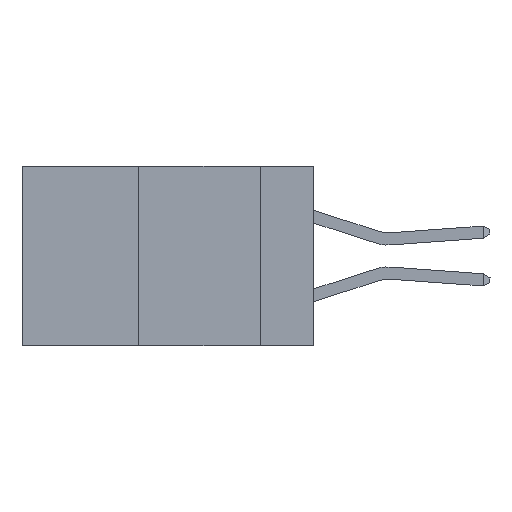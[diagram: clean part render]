
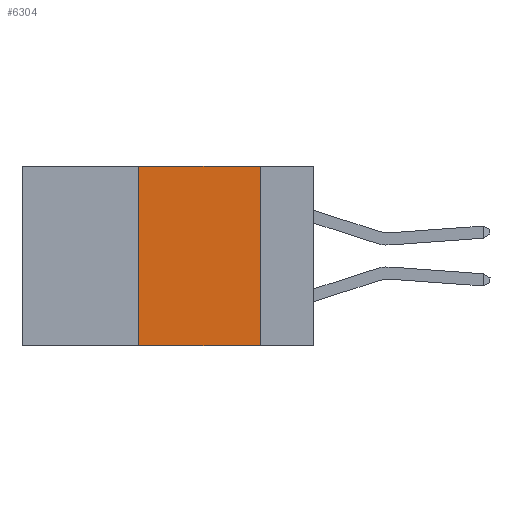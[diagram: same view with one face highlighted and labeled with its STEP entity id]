
A CAD part, left-side view. The second image highlights one B-rep face of the part: STEP entity #6304.
In plain terms, the highlighted planar face has unit normal (-1, 0, 0).
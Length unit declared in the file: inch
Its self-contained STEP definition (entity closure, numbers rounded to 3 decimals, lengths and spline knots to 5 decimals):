
#438 = DIRECTION ( 'NONE',  ( 0., -1., 0. ) ) ;
#831 = CARTESIAN_POINT ( 'NONE',  ( 0., 0.36, -0.37 ) ) ;
#860 = CARTESIAN_POINT ( 'NONE',  ( 0., 0.11, 0. ) ) ;
#1111 = CARTESIAN_POINT ( 'NONE',  ( 0., 0.36, 0. ) ) ;
#1325 = EDGE_CURVE ( 'NONE', #8755, #4644, #7580, .T. ) ;
#1890 = DIRECTION ( 'NONE',  ( 0., 0., 1. ) ) ;
#1956 = VECTOR ( 'NONE', #3213, 39.37008 ) ;
#1985 = CARTESIAN_POINT ( 'NONE',  ( 0., 0.6, -0.37 ) ) ;
#2091 = PLANE ( 'NONE',  #4279 ) ;
#2869 = LINE ( 'NONE', #1985, #8856 ) ;
#3213 = DIRECTION ( 'NONE',  ( 0., 0., -1. ) ) ;
#3431 = VECTOR ( 'NONE', #6434, 39.37008 ) ;
#3619 = ORIENTED_EDGE ( 'NONE', *, *, #7674, .F. ) ;
#3677 = DIRECTION ( 'NONE',  ( 0., 0., -1. ) ) ;
#3776 = CARTESIAN_POINT ( 'NONE',  ( 0., 0.11, 0. ) ) ;
#4201 = CARTESIAN_POINT ( 'NONE',  ( 0., 0.36, 0. ) ) ;
#4279 = AXIS2_PLACEMENT_3D ( 'NONE', #9880, #4387, #3677 ) ;
#4387 = DIRECTION ( 'NONE',  ( 1., 0., 0. ) ) ;
#4644 = VERTEX_POINT ( 'NONE', #1111 ) ;
#4693 = EDGE_CURVE ( 'NONE', #8755, #7034, #2869, .T. ) ;
#6079 = LINE ( 'NONE', #860, #1956 ) ;
#6304 = ADVANCED_FACE ( 'NONE', ( #8097 ), #2091, .F. ) ;
#6434 = DIRECTION ( 'NONE',  ( 0., -1., 0. ) ) ;
#7034 = VERTEX_POINT ( 'NONE', #9373 ) ;
#7105 = CARTESIAN_POINT ( 'NONE',  ( 0., 0.6, 0. ) ) ;
#7417 = EDGE_LOOP ( 'NONE', ( #9741, #3619, #7786, #8228 ) ) ;
#7464 = EDGE_CURVE ( 'NONE', #9459, #7034, #6079, .T. ) ;
#7580 = LINE ( 'NONE', #4201, #10023 ) ;
#7674 = EDGE_CURVE ( 'NONE', #4644, #9459, #8679, .T. ) ;
#7786 = ORIENTED_EDGE ( 'NONE', *, *, #1325, .F. ) ;
#8097 = FACE_OUTER_BOUND ( 'NONE', #7417, .T. ) ;
#8228 = ORIENTED_EDGE ( 'NONE', *, *, #4693, .T. ) ;
#8679 = LINE ( 'NONE', #7105, #3431 ) ;
#8755 = VERTEX_POINT ( 'NONE', #831 ) ;
#8856 = VECTOR ( 'NONE', #438, 39.37008 ) ;
#9373 = CARTESIAN_POINT ( 'NONE',  ( 0., 0.11, -0.37 ) ) ;
#9459 = VERTEX_POINT ( 'NONE', #3776 ) ;
#9741 = ORIENTED_EDGE ( 'NONE', *, *, #7464, .F. ) ;
#9880 = CARTESIAN_POINT ( 'NONE',  ( 0., 0.6, 0. ) ) ;
#10023 = VECTOR ( 'NONE', #1890, 39.37008 ) ;
